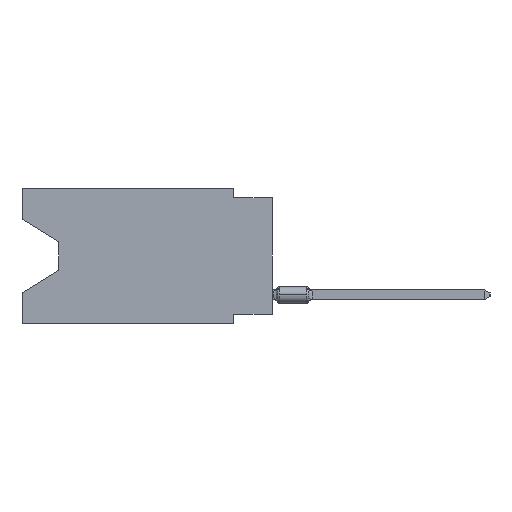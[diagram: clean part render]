
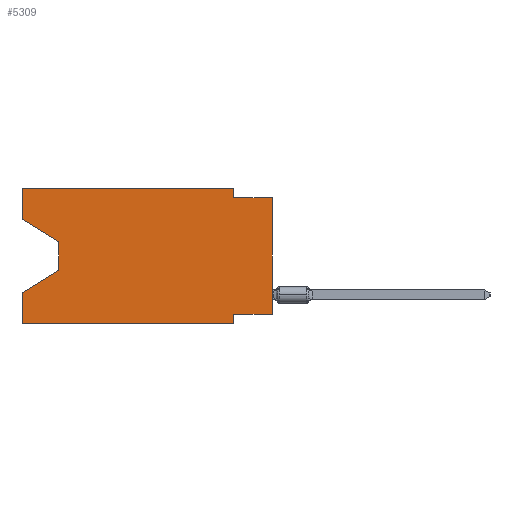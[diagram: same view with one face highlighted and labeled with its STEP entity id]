
A CAD part, left-side view. The second image highlights one B-rep face of the part: STEP entity #5309.
In plain terms, the highlighted planar face has unit normal (-1, 0, 0).
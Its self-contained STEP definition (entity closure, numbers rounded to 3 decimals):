
#2963 = VERTEX_POINT ( 'NONE', #44609 ) ;
#3396 = EDGE_CURVE ( 'NONE', #9700, #27385, #48569, .T. ) ;
#3560 = CARTESIAN_POINT ( 'NONE',  ( 0., 0., -8.255 ) ) ;
#4117 = DIRECTION ( 'NONE',  ( 0., -0.855, -0.519 ) ) ;
#4135 = VECTOR ( 'NONE', #40380, 1000. ) ;
#4854 = CARTESIAN_POINT ( 'NONE',  ( 0., 16.383, -8.89 ) ) ;
#5309 = ADVANCED_FACE ( 'NONE', ( #50891 ), #11551, .F. ) ;
#5356 = CARTESIAN_POINT ( 'NONE',  ( 0., 16.383, 0. ) ) ;
#5642 = LINE ( 'NONE', #5356, #32010 ) ;
#5692 = DIRECTION ( 'NONE',  ( 0., -1., 0. ) ) ;
#5756 = DIRECTION ( 'NONE',  ( 0., -1., 0. ) ) ;
#5918 = CARTESIAN_POINT ( 'NONE',  ( 0., 16.383, -2.038 ) ) ;
#6399 = DIRECTION ( 'NONE',  ( 0., 0., -1. ) ) ;
#9416 = CARTESIAN_POINT ( 'NONE',  ( 0., 0., -0.635 ) ) ;
#9700 = VERTEX_POINT ( 'NONE', #24058 ) ;
#11551 = PLANE ( 'NONE',  #44465 ) ;
#11921 = VECTOR ( 'NONE', #56686, 1000. ) ;
#11946 = CARTESIAN_POINT ( 'NONE',  ( 0., 2.54, 0. ) ) ;
#12432 = VECTOR ( 'NONE', #14124, 1000. ) ;
#13094 = DIRECTION ( 'NONE',  ( 0., 0., -1. ) ) ;
#13941 = CARTESIAN_POINT ( 'NONE',  ( 0., 0., 0. ) ) ;
#14101 = VERTEX_POINT ( 'NONE', #3560 ) ;
#14124 = DIRECTION ( 'NONE',  ( 0., 0.855, -0.519 ) ) ;
#14937 = ORIENTED_EDGE ( 'NONE', *, *, #48446, .F. ) ;
#15043 = CARTESIAN_POINT ( 'NONE',  ( 0., 0., -0.635 ) ) ;
#15395 = CARTESIAN_POINT ( 'NONE',  ( 0., 2.54, 0. ) ) ;
#15761 = EDGE_CURVE ( 'NONE', #22019, #9700, #22860, .T. ) ;
#16846 = DIRECTION ( 'NONE',  ( 0., -1., 0. ) ) ;
#17347 = CARTESIAN_POINT ( 'NONE',  ( 0., 16.383, -2.038 ) ) ;
#18261 = LINE ( 'NONE', #13941, #32572 ) ;
#18579 = EDGE_CURVE ( 'NONE', #14101, #54260, #29231, .T. ) ;
#18863 = VERTEX_POINT ( 'NONE', #15043 ) ;
#19112 = DIRECTION ( 'NONE',  ( 0., 0., 1. ) ) ;
#19228 = ORIENTED_EDGE ( 'NONE', *, *, #3396, .F. ) ;
#19334 = ORIENTED_EDGE ( 'NONE', *, *, #31226, .T. ) ;
#20273 = VERTEX_POINT ( 'NONE', #30671 ) ;
#21339 = VECTOR ( 'NONE', #5692, 1000. ) ;
#21738 = CARTESIAN_POINT ( 'NONE',  ( 0., 16.383, -8.89 ) ) ;
#22019 = VERTEX_POINT ( 'NONE', #5918 ) ;
#22860 = LINE ( 'NONE', #53300, #4135 ) ;
#23205 = VECTOR ( 'NONE', #5756, 1000. ) ;
#24007 = CARTESIAN_POINT ( 'NONE',  ( 0., 2.54, -8.89 ) ) ;
#24020 = LINE ( 'NONE', #15395, #29384 ) ;
#24058 = CARTESIAN_POINT ( 'NONE',  ( 0., 16.383, 0. ) ) ;
#25004 = ORIENTED_EDGE ( 'NONE', *, *, #48694, .T. ) ;
#26743 = CARTESIAN_POINT ( 'NONE',  ( 0., 13.97, -3.505 ) ) ;
#27385 = VERTEX_POINT ( 'NONE', #11946 ) ;
#27492 = EDGE_LOOP ( 'NONE', ( #40593, #52735, #29476, #31798, #25004, #37156, #47042, #19334, #14937, #29458, #19228, #29142 ) ) ;
#27595 = EDGE_CURVE ( 'NONE', #22019, #41359, #30817, .T. ) ;
#28592 = DIRECTION ( 'NONE',  ( 0., 0., -1. ) ) ;
#28934 = DIRECTION ( 'NONE',  ( 0., 1., 0. ) ) ;
#29089 = CARTESIAN_POINT ( 'NONE',  ( 0., 16.383, -6.852 ) ) ;
#29142 = ORIENTED_EDGE ( 'NONE', *, *, #15761, .F. ) ;
#29231 = LINE ( 'NONE', #55370, #54748 ) ;
#29241 = LINE ( 'NONE', #46203, #12432 ) ;
#29384 = VECTOR ( 'NONE', #28592, 1000. ) ;
#29458 = ORIENTED_EDGE ( 'NONE', *, *, #51973, .F. ) ;
#29476 = ORIENTED_EDGE ( 'NONE', *, *, #31607, .T. ) ;
#30671 = CARTESIAN_POINT ( 'NONE',  ( 0., 2.54, -0.635 ) ) ;
#30817 = LINE ( 'NONE', #17347, #47900 ) ;
#31226 = EDGE_CURVE ( 'NONE', #14101, #18863, #18261, .T. ) ;
#31607 = EDGE_CURVE ( 'NONE', #2963, #52394, #29241, .T. ) ;
#31798 = ORIENTED_EDGE ( 'NONE', *, *, #35260, .F. ) ;
#32010 = VECTOR ( 'NONE', #49594, 1000. ) ;
#32523 = DIRECTION ( 'NONE',  ( 1., 0., 0. ) ) ;
#32572 = VECTOR ( 'NONE', #19112, 1000. ) ;
#34870 = CARTESIAN_POINT ( 'NONE',  ( 0., 13.97, -3.505 ) ) ;
#35200 = LINE ( 'NONE', #47859, #44820 ) ;
#35260 = EDGE_CURVE ( 'NONE', #52983, #52394, #5642, .T. ) ;
#37156 = ORIENTED_EDGE ( 'NONE', *, *, #39240, .F. ) ;
#39240 = EDGE_CURVE ( 'NONE', #54260, #55773, #35200, .T. ) ;
#40380 = DIRECTION ( 'NONE',  ( 0., 0., 1. ) ) ;
#40593 = ORIENTED_EDGE ( 'NONE', *, *, #27595, .T. ) ;
#40646 = VECTOR ( 'NONE', #16846, 1000. ) ;
#41359 = VERTEX_POINT ( 'NONE', #26743 ) ;
#44346 = LINE ( 'NONE', #34870, #11921 ) ;
#44465 = AXIS2_PLACEMENT_3D ( 'NONE', #54359, #32523, #6399 ) ;
#44609 = CARTESIAN_POINT ( 'NONE',  ( 0., 13.97, -5.385 ) ) ;
#44820 = VECTOR ( 'NONE', #13094, 1000. ) ;
#46203 = CARTESIAN_POINT ( 'NONE',  ( 0., 13.97, -5.385 ) ) ;
#47042 = ORIENTED_EDGE ( 'NONE', *, *, #18579, .F. ) ;
#47859 = CARTESIAN_POINT ( 'NONE',  ( 0., 2.54, -8.89 ) ) ;
#47900 = VECTOR ( 'NONE', #4117, 1000. ) ;
#48446 = EDGE_CURVE ( 'NONE', #20273, #18863, #48778, .T. ) ;
#48569 = LINE ( 'NONE', #49135, #23205 ) ;
#48694 = EDGE_CURVE ( 'NONE', #52983, #55773, #55915, .T. ) ;
#48778 = LINE ( 'NONE', #9416, #21339 ) ;
#49135 = CARTESIAN_POINT ( 'NONE',  ( 0., 16.383, 0. ) ) ;
#49594 = DIRECTION ( 'NONE',  ( 0., 0., 1. ) ) ;
#50891 = FACE_OUTER_BOUND ( 'NONE', #27492, .T. ) ;
#51008 = EDGE_CURVE ( 'NONE', #41359, #2963, #44346, .T. ) ;
#51973 = EDGE_CURVE ( 'NONE', #27385, #20273, #24020, .T. ) ;
#52394 = VERTEX_POINT ( 'NONE', #29089 ) ;
#52556 = CARTESIAN_POINT ( 'NONE',  ( 0., 2.54, -8.255 ) ) ;
#52735 = ORIENTED_EDGE ( 'NONE', *, *, #51008, .T. ) ;
#52983 = VERTEX_POINT ( 'NONE', #4854 ) ;
#53300 = CARTESIAN_POINT ( 'NONE',  ( 0., 16.383, 0. ) ) ;
#54260 = VERTEX_POINT ( 'NONE', #52556 ) ;
#54359 = CARTESIAN_POINT ( 'NONE',  ( 0., 16.383, 0. ) ) ;
#54748 = VECTOR ( 'NONE', #28934, 1000. ) ;
#55370 = CARTESIAN_POINT ( 'NONE',  ( 0., 0., -8.255 ) ) ;
#55773 = VERTEX_POINT ( 'NONE', #24007 ) ;
#55915 = LINE ( 'NONE', #21738, #40646 ) ;
#56686 = DIRECTION ( 'NONE',  ( 0., 0., -1. ) ) ;
